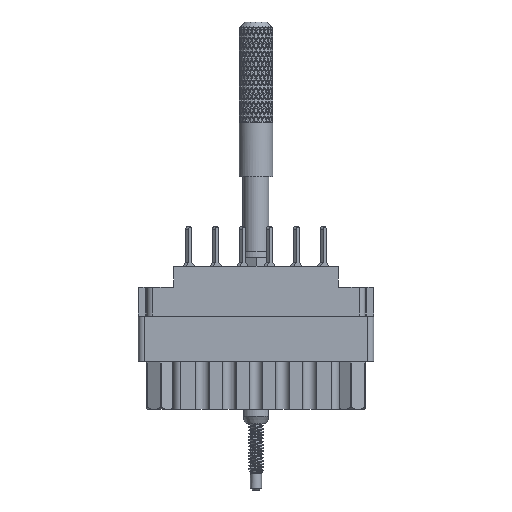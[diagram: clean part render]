
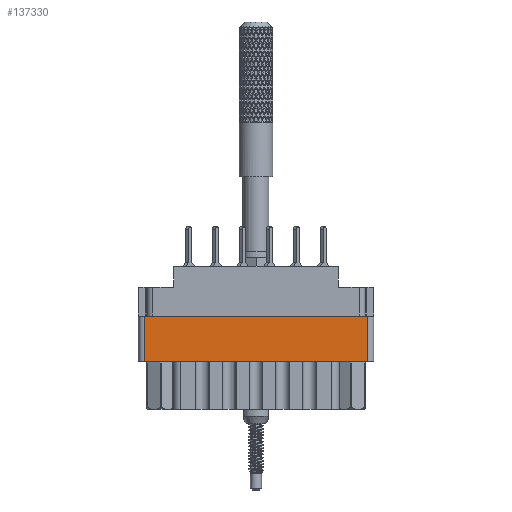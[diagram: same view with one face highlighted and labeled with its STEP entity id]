
A CAD part, front view. The second image highlights one B-rep face of the part: STEP entity #137330.
In plain terms, the highlighted planar face has unit normal (0, -1, 0).
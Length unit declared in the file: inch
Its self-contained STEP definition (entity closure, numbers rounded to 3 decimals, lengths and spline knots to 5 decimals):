
#340 = EDGE_CURVE ( 'NONE', #189890, #163940, #159244, .T. ) ;
#1589 = EDGE_CURVE ( 'NONE', #23688, #122506, #88297, .T. ) ;
#12064 = CARTESIAN_POINT ( 'NONE',  ( 0.624, -0.343, -0.529 ) ) ;
#12595 = CARTESIAN_POINT ( 'NONE',  ( -0.624, -0.343, -0.798 ) ) ;
#18660 = VECTOR ( 'NONE', #164033, 39.37008 ) ;
#23688 = VERTEX_POINT ( 'NONE', #12064 ) ;
#57205 = CARTESIAN_POINT ( 'NONE',  ( 0.624, -0.343, -0.529 ) ) ;
#58963 = ORIENTED_EDGE ( 'NONE', *, *, #1589, .F. ) ;
#66498 = ORIENTED_EDGE ( 'NONE', *, *, #340, .F. ) ;
#78146 = DIRECTION ( 'NONE',  ( 0., 0., 1. ) ) ;
#81189 = ORIENTED_EDGE ( 'NONE', *, *, #138152, .F. ) ;
#81698 = LINE ( 'NONE', #151910, #130644 ) ;
#88297 = LINE ( 'NONE', #57205, #18660 ) ;
#90269 = FACE_OUTER_BOUND ( 'NONE', #108258, .T. ) ;
#98688 = ORIENTED_EDGE ( 'NONE', *, *, #150470, .T. ) ;
#99260 = VECTOR ( 'NONE', #177627, 39.37008 ) ;
#108258 = EDGE_LOOP ( 'NONE', ( #81189, #58963, #98688, #66498 ) ) ;
#108983 = LINE ( 'NONE', #126418, #140736 ) ;
#116821 = CARTESIAN_POINT ( 'NONE',  ( -0.624, -0.343, -0.529 ) ) ;
#119419 = DIRECTION ( 'NONE',  ( 0., 0., -1. ) ) ;
#122506 = VERTEX_POINT ( 'NONE', #116821 ) ;
#122534 = CARTESIAN_POINT ( 'NONE',  ( 0.624, -0.343, -0.277 ) ) ;
#126418 = CARTESIAN_POINT ( 'NONE',  ( 0.624, -0.343, -0.798 ) ) ;
#127364 = DIRECTION ( 'NONE',  ( 0., 0., 1. ) ) ;
#130644 = VECTOR ( 'NONE', #78146, 39.37008 ) ;
#133700 = AXIS2_PLACEMENT_3D ( 'NONE', #12595, #147569, #119419 ) ;
#137330 = ADVANCED_FACE ( 'NONE', ( #90269 ), #145653, .T. ) ;
#138152 = EDGE_CURVE ( 'NONE', #122506, #189890, #81698, .T. ) ;
#140736 = VECTOR ( 'NONE', #127364, 39.37008 ) ;
#145653 = PLANE ( 'NONE',  #133700 ) ;
#147569 = DIRECTION ( 'NONE',  ( 0., -1., 0. ) ) ;
#150470 = EDGE_CURVE ( 'NONE', #23688, #163940, #108983, .T. ) ;
#151910 = CARTESIAN_POINT ( 'NONE',  ( -0.624, -0.343, -0.798 ) ) ;
#159244 = LINE ( 'NONE', #163072, #99260 ) ;
#163072 = CARTESIAN_POINT ( 'NONE',  ( -0.656, -0.343, -0.277 ) ) ;
#163940 = VERTEX_POINT ( 'NONE', #122534 ) ;
#164033 = DIRECTION ( 'NONE',  ( -1., 0., 0. ) ) ;
#175150 = CARTESIAN_POINT ( 'NONE',  ( -0.624, -0.343, -0.277 ) ) ;
#177627 = DIRECTION ( 'NONE',  ( 1., 0., 0. ) ) ;
#189890 = VERTEX_POINT ( 'NONE', #175150 ) ;
